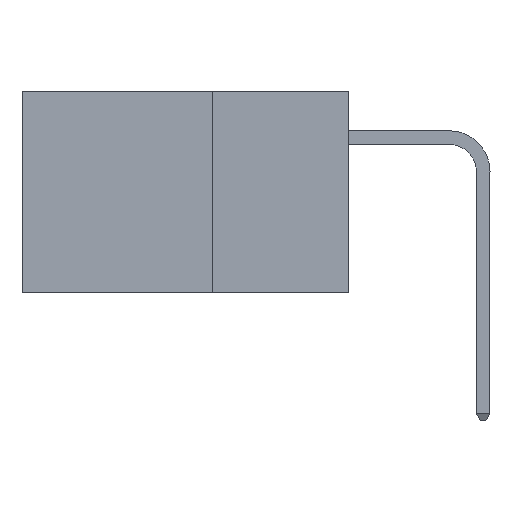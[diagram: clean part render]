
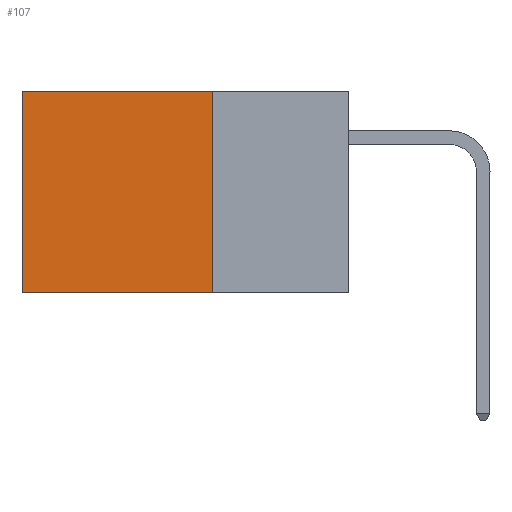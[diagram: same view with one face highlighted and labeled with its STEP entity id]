
A CAD part, left-side view. The second image highlights one B-rep face of the part: STEP entity #107.
In plain terms, the highlighted planar face has unit normal (-1, 0, 0).
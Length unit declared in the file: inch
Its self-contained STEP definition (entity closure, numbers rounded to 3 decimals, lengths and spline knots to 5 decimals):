
#107 = ADVANCED_FACE ( 'NONE', ( #5489 ), #2907, .F. ) ;
#259 = VECTOR ( 'NONE', #17630, 39.37008 ) ;
#556 = DIRECTION ( 'NONE',  ( 0., 0., -1. ) ) ;
#1662 = EDGE_LOOP ( 'NONE', ( #18550, #14676, #14729, #4660 ) ) ;
#1838 = DIRECTION ( 'NONE',  ( 0., 1., 0. ) ) ;
#2090 = CARTESIAN_POINT ( 'NONE',  ( 0.2875, 0.25, -0.37 ) ) ;
#2907 = PLANE ( 'NONE',  #20134 ) ;
#4660 = ORIENTED_EDGE ( 'NONE', *, *, #21023, .T. ) ;
#5317 = LINE ( 'NONE', #16057, #259 ) ;
#5489 = FACE_OUTER_BOUND ( 'NONE', #1662, .T. ) ;
#5945 = EDGE_CURVE ( 'NONE', #11969, #14667, #12776, .T. ) ;
#6150 = VERTEX_POINT ( 'NONE', #16271 ) ;
#7929 = DIRECTION ( 'NONE',  ( 0., 0., -1. ) ) ;
#8493 = VECTOR ( 'NONE', #1838, 39.37008 ) ;
#8647 = DIRECTION ( 'NONE',  ( 1., 0., 0. ) ) ;
#9549 = VECTOR ( 'NONE', #556, 39.37008 ) ;
#10473 = CARTESIAN_POINT ( 'NONE',  ( 0.2875, 0.25, -0.37 ) ) ;
#11118 = CARTESIAN_POINT ( 'NONE',  ( 0.2875, 0.25, 0. ) ) ;
#11969 = VERTEX_POINT ( 'NONE', #10473 ) ;
#12161 = CARTESIAN_POINT ( 'NONE',  ( 0.2875, 0.6, 0. ) ) ;
#12404 = LINE ( 'NONE', #11118, #13940 ) ;
#12776 = LINE ( 'NONE', #2090, #8493 ) ;
#12860 = CARTESIAN_POINT ( 'NONE',  ( 0.2875, 0.6, -0.37 ) ) ;
#13940 = VECTOR ( 'NONE', #20665, 39.37008 ) ;
#14458 = CARTESIAN_POINT ( 'NONE',  ( 0.2875, 0.6, 0. ) ) ;
#14667 = VERTEX_POINT ( 'NONE', #12860 ) ;
#14676 = ORIENTED_EDGE ( 'NONE', *, *, #5945, .F. ) ;
#14729 = ORIENTED_EDGE ( 'NONE', *, *, #18406, .F. ) ;
#15010 = CARTESIAN_POINT ( 'NONE',  ( 0.2875, 0.25, 0. ) ) ;
#16057 = CARTESIAN_POINT ( 'NONE',  ( 0.2875, 0.25, 0. ) ) ;
#16271 = CARTESIAN_POINT ( 'NONE',  ( 0.2875, 0.25, 0. ) ) ;
#17303 = VERTEX_POINT ( 'NONE', #14458 ) ;
#17630 = DIRECTION ( 'NONE',  ( 0., 1., 0. ) ) ;
#18406 = EDGE_CURVE ( 'NONE', #6150, #11969, #12404, .T. ) ;
#18550 = ORIENTED_EDGE ( 'NONE', *, *, #19479, .T. ) ;
#18603 = LINE ( 'NONE', #12161, #9549 ) ;
#19479 = EDGE_CURVE ( 'NONE', #17303, #14667, #18603, .T. ) ;
#20134 = AXIS2_PLACEMENT_3D ( 'NONE', #15010, #8647, #7929 ) ;
#20665 = DIRECTION ( 'NONE',  ( 0., 0., -1. ) ) ;
#21023 = EDGE_CURVE ( 'NONE', #6150, #17303, #5317, .T. ) ;
